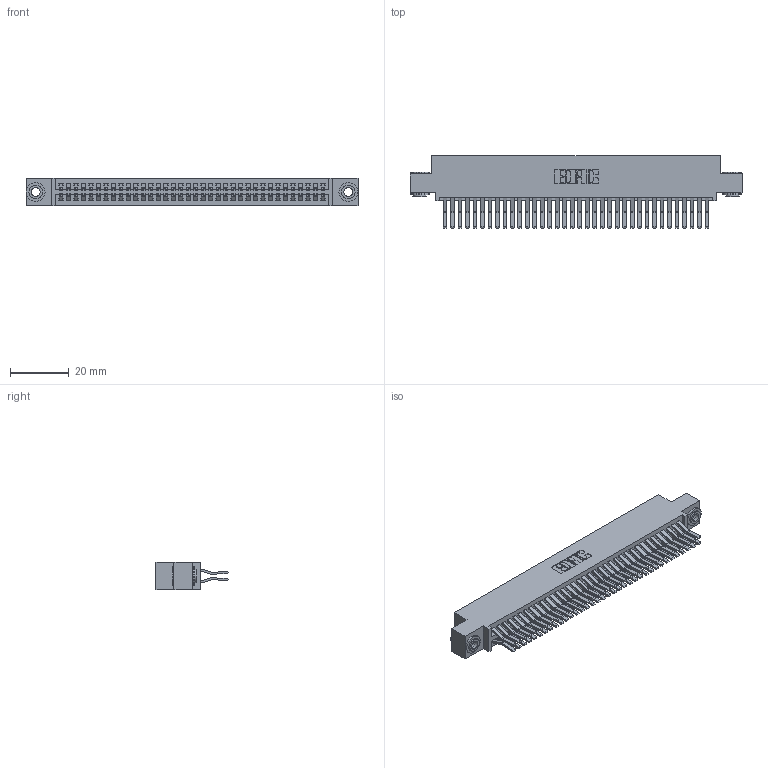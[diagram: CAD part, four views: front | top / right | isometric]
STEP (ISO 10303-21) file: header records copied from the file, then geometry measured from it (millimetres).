
FILE_DESCRIPTION (( 'STEP AP203' ), '1' );
FILE_NAME ('345-072-560-503.STEP', '2018-10-02T10:35:43', ( '' ), ( '' ), 'SwSTEP 2.0', 'SolidWorks 2016', '' );
FILE_SCHEMA (( 'CONFIG_CONTROL_DESIGN' ));
Length unit declared in the file: inch
Products named in the file (4): 345 Part_0.110 Offset - 0.156 Dia-TH; 345-072-560-503; 345-250-002_345-250-002-102; 345-292-001_560 Tail
Assembly tree (75 placements, depth 2):
  345-072-560-503
    345 Part_0.110 Offset - 0.156 Dia-TH
    345-292-001_560 Tail  x72
    345-250-002_345-250-002-102  x2
Bounding box: 112.65 x 24.45 x 9.4 mm (x, y, z)
Volume: 11305.1 mm3; surface area: 18106.1 mm2
Topology: 75 solids, 75 shells, 3912 faces, 11589 edges, 7626 vertices
Faces by surface type: plane 2470, cylinder 1434, cone 8
Entity records: 29924 total; most frequent: CARTESIAN_POINT 4999, ORIENTED_EDGE 4926, DIRECTION 4449, EDGE_CURVE 2463, VECTOR 2159, LINE 2159, VERTEX_POINT 1638, AXIS2_PLACEMENT_3D 1145
